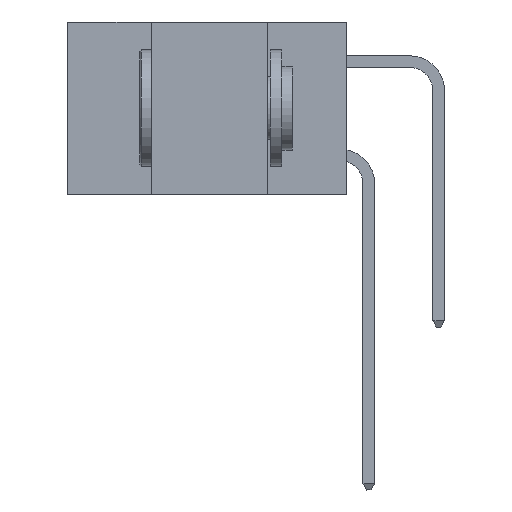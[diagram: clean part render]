
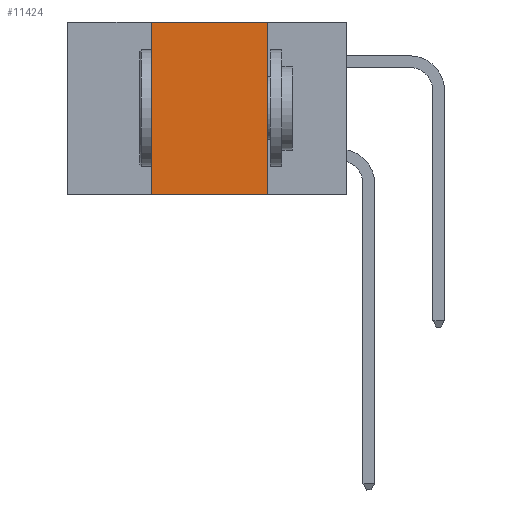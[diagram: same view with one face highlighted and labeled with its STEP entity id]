
A CAD part, left-side view. The second image highlights one B-rep face of the part: STEP entity #11424.
In plain terms, the highlighted planar face has unit normal (-1, 0, 0).
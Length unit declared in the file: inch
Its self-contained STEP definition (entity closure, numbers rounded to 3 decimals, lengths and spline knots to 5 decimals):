
#471 = ORIENTED_EDGE ( 'NONE', *, *, #7071, .F. ) ;
#891 = VERTEX_POINT ( 'NONE', #6272 ) ;
#1311 = CARTESIAN_POINT ( 'NONE',  ( 0., 0.42, 0. ) ) ;
#1985 = CARTESIAN_POINT ( 'NONE',  ( 0., 0.17, 0. ) ) ;
#2147 = ORIENTED_EDGE ( 'NONE', *, *, #24089, .F. ) ;
#4294 = PLANE ( 'NONE',  #16975 ) ;
#4929 = VECTOR ( 'NONE', #9797, 39.37008 ) ;
#6050 = DIRECTION ( 'NONE',  ( 0., 0., -1. ) ) ;
#6272 = CARTESIAN_POINT ( 'NONE',  ( 0., 0.42, -0.37 ) ) ;
#7071 = EDGE_CURVE ( 'NONE', #23106, #25383, #14464, .T. ) ;
#8006 = VECTOR ( 'NONE', #15857, 39.37008 ) ;
#8198 = VECTOR ( 'NONE', #14493, 39.37008 ) ;
#8958 = CARTESIAN_POINT ( 'NONE',  ( 0., 0.17, 0. ) ) ;
#9797 = DIRECTION ( 'NONE',  ( 0., -1., 0. ) ) ;
#10420 = CARTESIAN_POINT ( 'NONE',  ( 0., 0.17, -0.37 ) ) ;
#11424 = ADVANCED_FACE ( 'NONE', ( #18625 ), #4294, .F. ) ;
#11544 = EDGE_CURVE ( 'NONE', #891, #25383, #22311, .T. ) ;
#13455 = LINE ( 'NONE', #14764, #8198 ) ;
#13545 = DIRECTION ( 'NONE',  ( 0., 0., -1. ) ) ;
#13832 = CARTESIAN_POINT ( 'NONE',  ( 0., 0.42, 0. ) ) ;
#14464 = LINE ( 'NONE', #1985, #18535 ) ;
#14493 = DIRECTION ( 'NONE',  ( 0., -1., 0. ) ) ;
#14764 = CARTESIAN_POINT ( 'NONE',  ( 0., 0.6, 0. ) ) ;
#15799 = CARTESIAN_POINT ( 'NONE',  ( 0., 0.6, -0.37 ) ) ;
#15857 = DIRECTION ( 'NONE',  ( 0., 0., 1. ) ) ;
#16308 = ORIENTED_EDGE ( 'NONE', *, *, #19189, .F. ) ;
#16975 = AXIS2_PLACEMENT_3D ( 'NONE', #22440, #17439, #13545 ) ;
#17387 = EDGE_LOOP ( 'NONE', ( #471, #2147, #16308, #17812 ) ) ;
#17439 = DIRECTION ( 'NONE',  ( 1., 0., 0. ) ) ;
#17812 = ORIENTED_EDGE ( 'NONE', *, *, #11544, .T. ) ;
#18535 = VECTOR ( 'NONE', #6050, 39.37008 ) ;
#18625 = FACE_OUTER_BOUND ( 'NONE', #17387, .T. ) ;
#19189 = EDGE_CURVE ( 'NONE', #891, #23359, #21983, .T. ) ;
#21983 = LINE ( 'NONE', #13832, #8006 ) ;
#22311 = LINE ( 'NONE', #15799, #4929 ) ;
#22440 = CARTESIAN_POINT ( 'NONE',  ( 0., 0.6, 0. ) ) ;
#23106 = VERTEX_POINT ( 'NONE', #8958 ) ;
#23359 = VERTEX_POINT ( 'NONE', #1311 ) ;
#24089 = EDGE_CURVE ( 'NONE', #23359, #23106, #13455, .T. ) ;
#25383 = VERTEX_POINT ( 'NONE', #10420 ) ;
